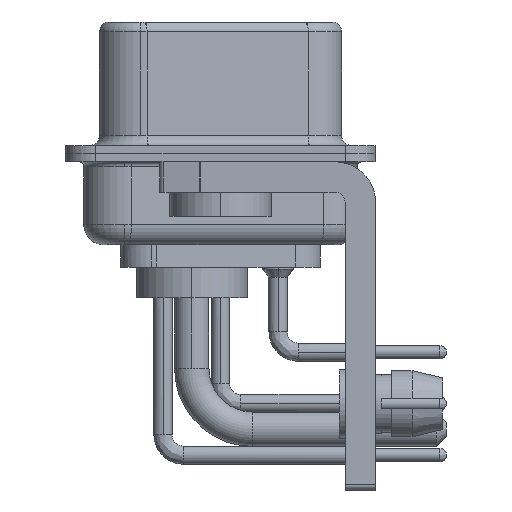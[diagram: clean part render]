
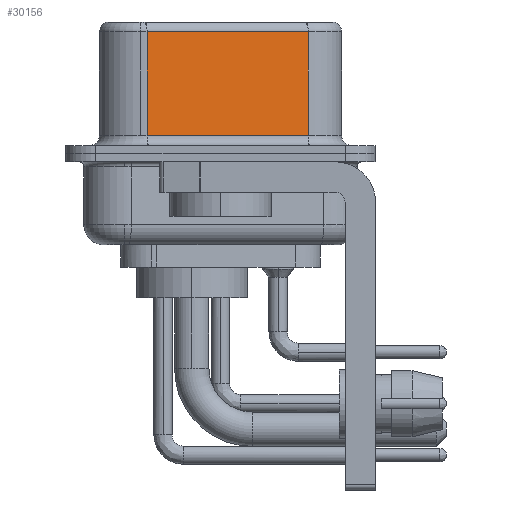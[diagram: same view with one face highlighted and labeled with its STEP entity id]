
A CAD part, left-side view. The second image highlights one B-rep face of the part: STEP entity #30156.
In plain terms, the highlighted planar face has unit normal (-0.985, -0.174, 0).
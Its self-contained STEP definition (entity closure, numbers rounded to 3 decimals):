
#449 = FACE_OUTER_BOUND ( 'NONE', #22714, .T. ) ;
#702 = CARTESIAN_POINT ( 'NONE',  ( 5.132, -4.322, 0.9 ) ) ;
#1689 = LINE ( 'NONE', #35928, #26435 ) ;
#2884 = DIRECTION ( 'NONE',  ( 0.985, 0.174, 0. ) ) ;
#3181 = DIRECTION ( 'NONE',  ( -0.174, 0.985, 0. ) ) ;
#3589 = DIRECTION ( 'NONE',  ( 0., 0., -1. ) ) ;
#3617 = DIRECTION ( 'NONE',  ( -0.174, 0.985, 0. ) ) ;
#3918 = CARTESIAN_POINT ( 'NONE',  ( 3.73, 3.628, 0.9 ) ) ;
#3990 = CARTESIAN_POINT ( 'NONE',  ( 5.132, -4.322, 0.9 ) ) ;
#4308 = DIRECTION ( 'NONE',  ( 0., 0., -1. ) ) ;
#6497 = EDGE_CURVE ( 'NONE', #25098, #10639, #22929, .T. ) ;
#6599 = VECTOR ( 'NONE', #3181, 1000. ) ;
#9024 = CARTESIAN_POINT ( 'NONE',  ( 5.132, -4.322, 6.52 ) ) ;
#10639 = VERTEX_POINT ( 'NONE', #30734 ) ;
#10720 = VERTEX_POINT ( 'NONE', #702 ) ;
#13523 = ORIENTED_EDGE ( 'NONE', *, *, #17364, .F. ) ;
#16207 = CARTESIAN_POINT ( 'NONE',  ( 5.132, -4.322, 6.02 ) ) ;
#17310 = VECTOR ( 'NONE', #31752, 1000. ) ;
#17364 = EDGE_CURVE ( 'NONE', #25098, #10720, #29114, .T. ) ;
#17557 = VECTOR ( 'NONE', #3589, 1000. ) ;
#20228 = ORIENTED_EDGE ( 'NONE', *, *, #6497, .T. ) ;
#21369 = ORIENTED_EDGE ( 'NONE', *, *, #24491, .T. ) ;
#22714 = EDGE_LOOP ( 'NONE', ( #13523, #20228, #27717, #21369 ) ) ;
#22883 = AXIS2_PLACEMENT_3D ( 'NONE', #9024, #2884, #3617 ) ;
#22929 = LINE ( 'NONE', #23120, #6599 ) ;
#23120 = CARTESIAN_POINT ( 'NONE',  ( 5.132, -4.322, 6.02 ) ) ;
#23553 = LINE ( 'NONE', #3990, #17310 ) ;
#24491 = EDGE_CURVE ( 'NONE', #26332, #10720, #23553, .T. ) ;
#25098 = VERTEX_POINT ( 'NONE', #16207 ) ;
#26332 = VERTEX_POINT ( 'NONE', #3918 ) ;
#26435 = VECTOR ( 'NONE', #4308, 1000. ) ;
#27717 = ORIENTED_EDGE ( 'NONE', *, *, #29586, .T. ) ;
#29114 = LINE ( 'NONE', #30669, #17557 ) ;
#29586 = EDGE_CURVE ( 'NONE', #10639, #26332, #1689, .T. ) ;
#30156 = ADVANCED_FACE ( 'NONE', ( #449 ), #31750, .F. ) ;
#30669 = CARTESIAN_POINT ( 'NONE',  ( 5.132, -4.322, 6.52 ) ) ;
#30734 = CARTESIAN_POINT ( 'NONE',  ( 3.73, 3.628, 6.02 ) ) ;
#31750 = PLANE ( 'NONE',  #22883 ) ;
#31752 = DIRECTION ( 'NONE',  ( 0.174, -0.985, 0. ) ) ;
#35928 = CARTESIAN_POINT ( 'NONE',  ( 3.73, 3.628, 6.52 ) ) ;
